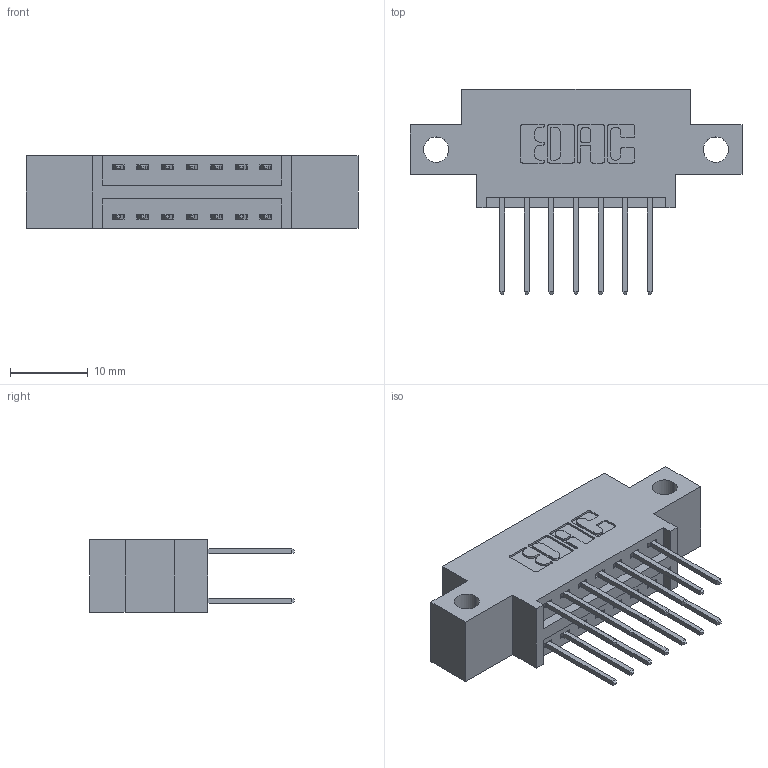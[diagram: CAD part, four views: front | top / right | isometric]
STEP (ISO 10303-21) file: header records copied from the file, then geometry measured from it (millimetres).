
FILE_DESCRIPTION (( 'STEP AP203' ), '1' );
FILE_NAME ('396-014-522-812.STEP', '2018-08-31T09:38:24', ( '' ), ( '' ), 'SwSTEP 2.0', 'SolidWorks 2016', '' );
FILE_SCHEMA (( 'CONFIG_CONTROL_DESIGN' ));
Length unit declared in the file: inch
Products named in the file (3): 396-014-522-812; 346 Part_0.170 Offset - Side Mount; 345-292-001_345-293-122
Assembly tree (15 placements, depth 2):
  396-014-522-812
    346 Part_0.170 Offset - Side Mount
    345-292-001_345-293-122  x14
Bounding box: 42.8 x 26.42 x 9.4 mm (x, y, z)
Volume: 3695.6 mm3; surface area: 4738.2 mm2
Topology: 15 solids, 15 shells, 854 faces, 2511 edges, 1654 vertices
Faces by surface type: plane 570, cylinder 284
Entity records: 9433 total; most frequent: CARTESIAN_POINT 1604, ORIENTED_EDGE 1538, DIRECTION 1465, EDGE_CURVE 769, LINE 609, VECTOR 609, VERTEX_POINT 510, AXIS2_PLACEMENT_3D 428
